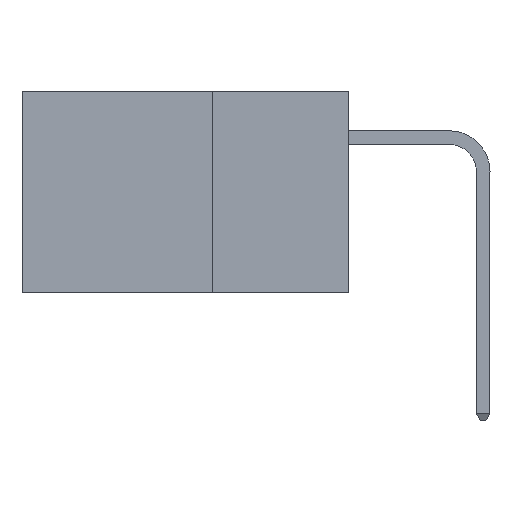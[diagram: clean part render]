
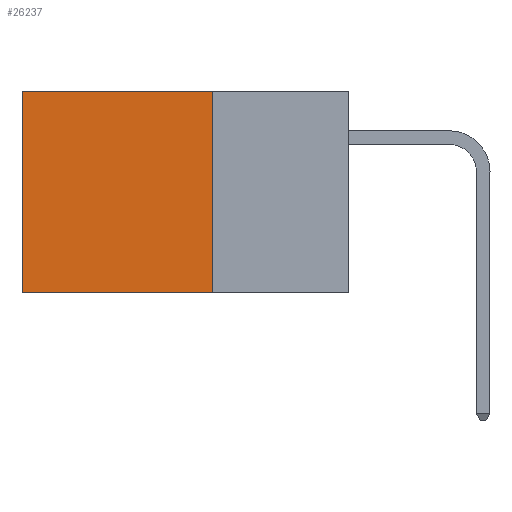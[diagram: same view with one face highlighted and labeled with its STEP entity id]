
A CAD part, left-side view. The second image highlights one B-rep face of the part: STEP entity #26237.
In plain terms, the highlighted planar face has unit normal (-1, 0, 0).
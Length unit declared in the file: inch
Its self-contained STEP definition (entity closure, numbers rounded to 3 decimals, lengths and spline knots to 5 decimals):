
#786 = VERTEX_POINT ( 'NONE', #27702 ) ;
#2292 = AXIS2_PLACEMENT_3D ( 'NONE', #29845, #14691, #32353 ) ;
#5431 = ORIENTED_EDGE ( 'NONE', *, *, #12571, .T. ) ;
#6940 = EDGE_LOOP ( 'NONE', ( #5431, #27530, #30694, #10082 ) ) ;
#8695 = DIRECTION ( 'NONE',  ( 0., 1., 0. ) ) ;
#9507 = PLANE ( 'NONE',  #2292 ) ;
#10004 = CARTESIAN_POINT ( 'NONE',  ( 0.2875, 0.25, -0.37 ) ) ;
#10082 = ORIENTED_EDGE ( 'NONE', *, *, #21469, .T. ) ;
#10834 = CARTESIAN_POINT ( 'NONE',  ( 0.2875, 0.25, 0. ) ) ;
#11618 = DIRECTION ( 'NONE',  ( 0., 0., -1. ) ) ;
#12188 = DIRECTION ( 'NONE',  ( 0., 0., -1. ) ) ;
#12571 = EDGE_CURVE ( 'NONE', #786, #16586, #13072, .T. ) ;
#13072 = LINE ( 'NONE', #22413, #25832 ) ;
#13321 = EDGE_CURVE ( 'NONE', #17063, #16586, #29678, .T. ) ;
#13516 = VECTOR ( 'NONE', #11618, 39.37008 ) ;
#14296 = FACE_OUTER_BOUND ( 'NONE', #6940, .T. ) ;
#14324 = LINE ( 'NONE', #16822, #13516 ) ;
#14691 = DIRECTION ( 'NONE',  ( 1., 0., 0. ) ) ;
#15994 = CARTESIAN_POINT ( 'NONE',  ( 0.2875, 0.6, -0.37 ) ) ;
#16586 = VERTEX_POINT ( 'NONE', #15994 ) ;
#16822 = CARTESIAN_POINT ( 'NONE',  ( 0.2875, 0.25, 0. ) ) ;
#17063 = VERTEX_POINT ( 'NONE', #28035 ) ;
#20857 = LINE ( 'NONE', #28869, #27512 ) ;
#21469 = EDGE_CURVE ( 'NONE', #30921, #786, #20857, .T. ) ;
#22413 = CARTESIAN_POINT ( 'NONE',  ( 0.2875, 0.6, 0. ) ) ;
#23043 = VECTOR ( 'NONE', #30311, 39.37008 ) ;
#25832 = VECTOR ( 'NONE', #12188, 39.37008 ) ;
#25833 = EDGE_CURVE ( 'NONE', #30921, #17063, #14324, .T. ) ;
#26237 = ADVANCED_FACE ( 'NONE', ( #14296 ), #9507, .F. ) ;
#27512 = VECTOR ( 'NONE', #8695, 39.37008 ) ;
#27530 = ORIENTED_EDGE ( 'NONE', *, *, #13321, .F. ) ;
#27702 = CARTESIAN_POINT ( 'NONE',  ( 0.2875, 0.6, 0. ) ) ;
#28035 = CARTESIAN_POINT ( 'NONE',  ( 0.2875, 0.25, -0.37 ) ) ;
#28869 = CARTESIAN_POINT ( 'NONE',  ( 0.2875, 0.25, 0. ) ) ;
#29678 = LINE ( 'NONE', #10004, #23043 ) ;
#29845 = CARTESIAN_POINT ( 'NONE',  ( 0.2875, 0.25, 0. ) ) ;
#30311 = DIRECTION ( 'NONE',  ( 0., 1., 0. ) ) ;
#30694 = ORIENTED_EDGE ( 'NONE', *, *, #25833, .F. ) ;
#30921 = VERTEX_POINT ( 'NONE', #10834 ) ;
#32353 = DIRECTION ( 'NONE',  ( 0., 0., -1. ) ) ;
